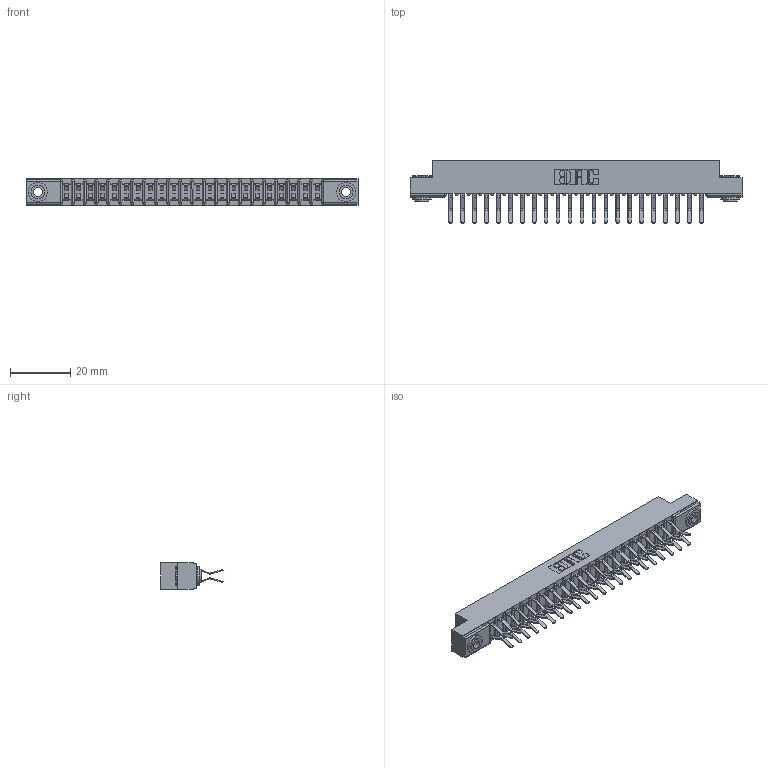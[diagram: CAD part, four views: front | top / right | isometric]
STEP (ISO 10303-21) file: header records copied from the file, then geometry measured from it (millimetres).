
FILE_DESCRIPTION (( 'STEP AP203' ), '1' );
FILE_NAME ('307-044-560-203.STEP', '2019-09-06T08:13:19', ( '' ), ( '' ), 'SwSTEP 2.0', 'SolidWorks 2016', '' );
FILE_SCHEMA (( 'CONFIG_CONTROL_DESIGN' ));
Length unit declared in the file: inch
Products named in the file (4): 345-250-002_345-250-002-102; 307 Part_.156 Dia Mounting Holes; 307-290-001_560; 307-044-560-203
Assembly tree (47 placements, depth 2):
  307-044-560-203
    307 Part_.156 Dia Mounting Holes
    307-290-001_560  x44
    345-250-002_345-250-002-102  x2
Bounding box: 110.19 x 20.73 x 8.71 mm (x, y, z)
Volume: 7263.4 mm3; surface area: 13409.4 mm2
Topology: 47 solids, 47 shells, 2393 faces, 6683 edges, 4330 vertices
Faces by surface type: plane 1546, cylinder 793, sphere 46, cone 8
Entity records: 23199 total; most frequent: CARTESIAN_POINT 3783, ORIENTED_EDGE 3738, DIRECTION 3729, EDGE_CURVE 1869, VECTOR 1417, LINE 1417, VERTEX_POINT 1210, AXIS2_PLACEMENT_3D 1156
